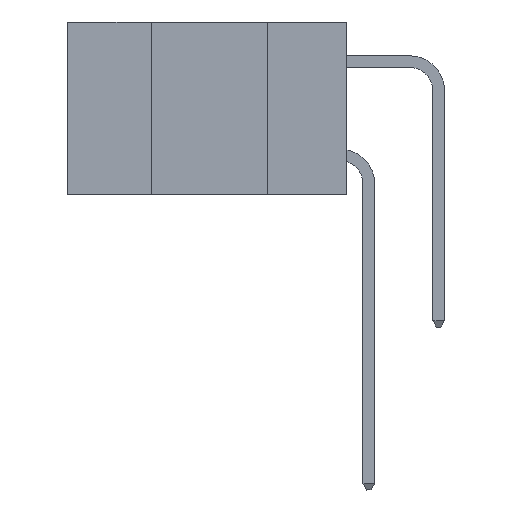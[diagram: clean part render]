
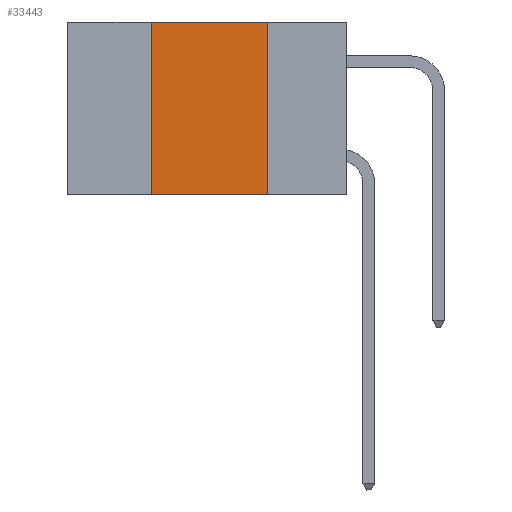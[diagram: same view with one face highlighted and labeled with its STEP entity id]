
A CAD part, left-side view. The second image highlights one B-rep face of the part: STEP entity #33443.
In plain terms, the highlighted planar face has unit normal (-1, 0, 0).
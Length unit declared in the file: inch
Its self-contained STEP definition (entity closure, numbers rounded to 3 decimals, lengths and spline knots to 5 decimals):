
#65 = CARTESIAN_POINT ( 'NONE',  ( 0., 0.6, 0. ) ) ;
#753 = DIRECTION ( 'NONE',  ( 0., 0., 1. ) ) ;
#786 = FACE_OUTER_BOUND ( 'NONE', #11491, .T. ) ;
#2923 = LINE ( 'NONE', #3282, #4580 ) ;
#3220 = CARTESIAN_POINT ( 'NONE',  ( 0., 0.6, -0.37 ) ) ;
#3282 = CARTESIAN_POINT ( 'NONE',  ( 0., 0.6, 0. ) ) ;
#3896 = ORIENTED_EDGE ( 'NONE', *, *, #14339, .F. ) ;
#4580 = VECTOR ( 'NONE', #8836, 39.37008 ) ;
#5520 = VERTEX_POINT ( 'NONE', #34575 ) ;
#7845 = EDGE_CURVE ( 'NONE', #30360, #25992, #31060, .T. ) ;
#8466 = ORIENTED_EDGE ( 'NONE', *, *, #15481, .F. ) ;
#8577 = DIRECTION ( 'NONE',  ( 0., 0., -1. ) ) ;
#8836 = DIRECTION ( 'NONE',  ( 0., -1., 0. ) ) ;
#9266 = DIRECTION ( 'NONE',  ( 0., 0., -1. ) ) ;
#9626 = ORIENTED_EDGE ( 'NONE', *, *, #7845, .F. ) ;
#11491 = EDGE_LOOP ( 'NONE', ( #3896, #8466, #9626, #12907 ) ) ;
#12215 = CARTESIAN_POINT ( 'NONE',  ( 0., 0.17, 0. ) ) ;
#12907 = ORIENTED_EDGE ( 'NONE', *, *, #18955, .T. ) ;
#13205 = CARTESIAN_POINT ( 'NONE',  ( 0., 0.42, -0.37 ) ) ;
#14339 = EDGE_CURVE ( 'NONE', #21038, #5520, #17940, .T. ) ;
#15481 = EDGE_CURVE ( 'NONE', #25992, #21038, #2923, .T. ) ;
#17940 = LINE ( 'NONE', #12215, #26354 ) ;
#18955 = EDGE_CURVE ( 'NONE', #30360, #5520, #25385, .T. ) ;
#19059 = CARTESIAN_POINT ( 'NONE',  ( 0., 0.17, 0. ) ) ;
#19847 = DIRECTION ( 'NONE',  ( 0., -1., 0. ) ) ;
#21038 = VERTEX_POINT ( 'NONE', #19059 ) ;
#24382 = VECTOR ( 'NONE', #753, 39.37008 ) ;
#25385 = LINE ( 'NONE', #3220, #29440 ) ;
#25992 = VERTEX_POINT ( 'NONE', #26155 ) ;
#26155 = CARTESIAN_POINT ( 'NONE',  ( 0., 0.42, 0. ) ) ;
#26354 = VECTOR ( 'NONE', #9266, 39.37008 ) ;
#28115 = CARTESIAN_POINT ( 'NONE',  ( 0., 0.42, 0. ) ) ;
#28512 = DIRECTION ( 'NONE',  ( 1., 0., 0. ) ) ;
#28693 = PLANE ( 'NONE',  #33011 ) ;
#29440 = VECTOR ( 'NONE', #19847, 39.37008 ) ;
#30360 = VERTEX_POINT ( 'NONE', #13205 ) ;
#31060 = LINE ( 'NONE', #28115, #24382 ) ;
#33011 = AXIS2_PLACEMENT_3D ( 'NONE', #65, #28512, #8577 ) ;
#33443 = ADVANCED_FACE ( 'NONE', ( #786 ), #28693, .F. ) ;
#34575 = CARTESIAN_POINT ( 'NONE',  ( 0., 0.17, -0.37 ) ) ;
